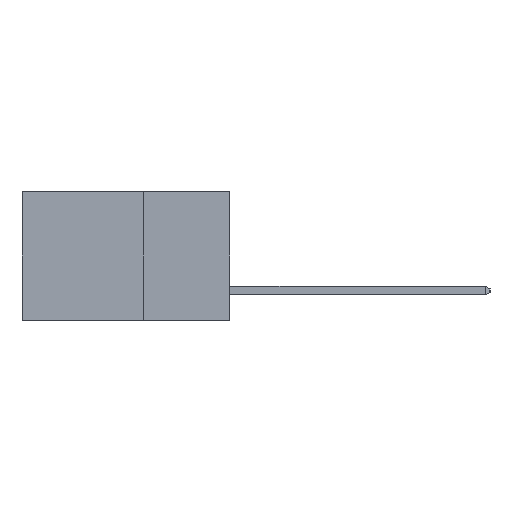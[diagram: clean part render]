
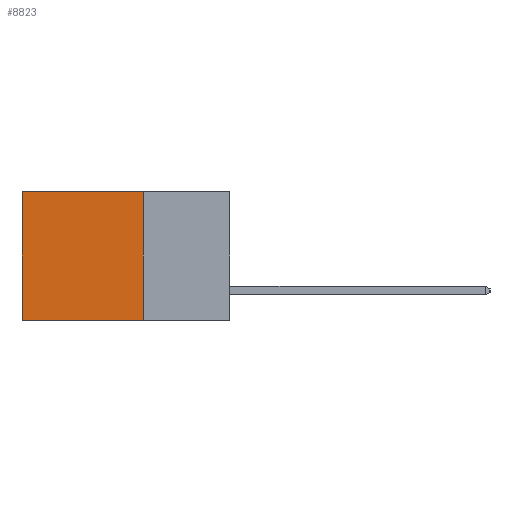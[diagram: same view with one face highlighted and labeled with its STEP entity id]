
A CAD part, left-side view. The second image highlights one B-rep face of the part: STEP entity #8823.
In plain terms, the highlighted planar face has unit normal (-1, 0, 0).
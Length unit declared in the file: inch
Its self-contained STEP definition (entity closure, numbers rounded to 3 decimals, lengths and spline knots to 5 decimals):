
#21 = ORIENTED_EDGE ( 'NONE', *, *, #961, .T. ) ;
#305 = CARTESIAN_POINT ( 'NONE',  ( 0.298, 0.25, -0.37 ) ) ;
#769 = VERTEX_POINT ( 'NONE', #11022 ) ;
#961 = EDGE_CURVE ( 'NONE', #3580, #1670, #8679, .T. ) ;
#1257 = CARTESIAN_POINT ( 'NONE',  ( 0.298, 0.25, 0. ) ) ;
#1670 = VERTEX_POINT ( 'NONE', #3686 ) ;
#2732 = CARTESIAN_POINT ( 'NONE',  ( 0.298, 0.25, 0. ) ) ;
#3580 = VERTEX_POINT ( 'NONE', #2732 ) ;
#3686 = CARTESIAN_POINT ( 'NONE',  ( 0.298, 0.6, 0. ) ) ;
#5118 = CARTESIAN_POINT ( 'NONE',  ( 0.298, 0.25, 0. ) ) ;
#5379 = VECTOR ( 'NONE', #8833, 39.37008 ) ;
#5711 = LINE ( 'NONE', #305, #5379 ) ;
#5893 = EDGE_CURVE ( 'NONE', #3580, #12757, #12046, .T. ) ;
#6178 = DIRECTION ( 'NONE',  ( 1., 0., 0. ) ) ;
#6194 = VECTOR ( 'NONE', #12863, 39.37008 ) ;
#6448 = FACE_OUTER_BOUND ( 'NONE', #11323, .T. ) ;
#6741 = ORIENTED_EDGE ( 'NONE', *, *, #13116, .F. ) ;
#6745 = EDGE_CURVE ( 'NONE', #1670, #769, #11012, .T. ) ;
#7366 = ORIENTED_EDGE ( 'NONE', *, *, #6745, .T. ) ;
#7773 = CARTESIAN_POINT ( 'NONE',  ( 0.298, 0.6, 0. ) ) ;
#8128 = VECTOR ( 'NONE', #9996, 39.37008 ) ;
#8679 = LINE ( 'NONE', #10506, #6194 ) ;
#8823 = ADVANCED_FACE ( 'NONE', ( #6448 ), #11523, .F. ) ;
#8833 = DIRECTION ( 'NONE',  ( 0., 1., 0. ) ) ;
#9770 = AXIS2_PLACEMENT_3D ( 'NONE', #5118, #6178, #13622 ) ;
#9996 = DIRECTION ( 'NONE',  ( 0., 0., -1. ) ) ;
#10506 = CARTESIAN_POINT ( 'NONE',  ( 0.298, 0.25, 0. ) ) ;
#11012 = LINE ( 'NONE', #7773, #8128 ) ;
#11022 = CARTESIAN_POINT ( 'NONE',  ( 0.298, 0.6, -0.37 ) ) ;
#11323 = EDGE_LOOP ( 'NONE', ( #7366, #6741, #11373, #21 ) ) ;
#11367 = VECTOR ( 'NONE', #11948, 39.37008 ) ;
#11373 = ORIENTED_EDGE ( 'NONE', *, *, #5893, .F. ) ;
#11523 = PLANE ( 'NONE',  #9770 ) ;
#11948 = DIRECTION ( 'NONE',  ( 0., 0., -1. ) ) ;
#12046 = LINE ( 'NONE', #1257, #11367 ) ;
#12757 = VERTEX_POINT ( 'NONE', #13413 ) ;
#12863 = DIRECTION ( 'NONE',  ( 0., 1., 0. ) ) ;
#13116 = EDGE_CURVE ( 'NONE', #12757, #769, #5711, .T. ) ;
#13413 = CARTESIAN_POINT ( 'NONE',  ( 0.298, 0.25, -0.37 ) ) ;
#13622 = DIRECTION ( 'NONE',  ( 0., 0., -1. ) ) ;
